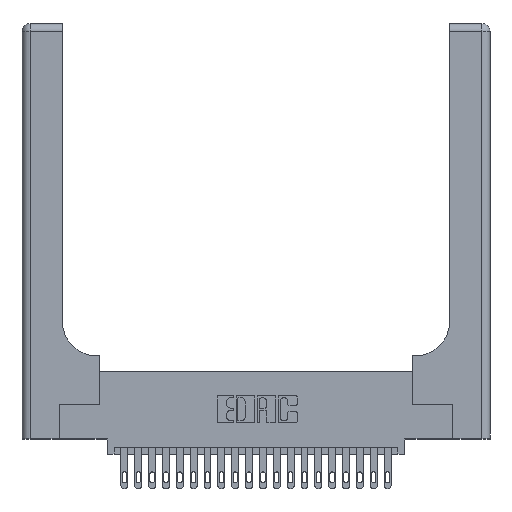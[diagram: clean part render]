
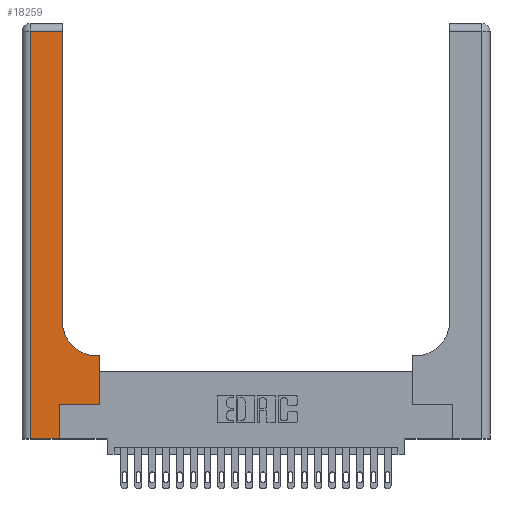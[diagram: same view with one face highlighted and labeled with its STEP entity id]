
A CAD part, top view. The second image highlights one B-rep face of the part: STEP entity #18259.
In plain terms, the highlighted planar face has unit normal (0, 0, 1).
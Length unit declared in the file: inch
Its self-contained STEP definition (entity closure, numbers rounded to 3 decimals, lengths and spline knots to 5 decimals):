
#500 = ORIENTED_EDGE ( 'NONE', *, *, #10486, .T. ) ;
#1205 = CIRCLE ( 'NONE', #1268, 0.25 ) ;
#1268 = AXIS2_PLACEMENT_3D ( 'NONE', #23259, #3258, #17698 ) ;
#1542 = EDGE_CURVE ( 'NONE', #22544, #12693, #17768, .T. ) ;
#1891 = ORIENTED_EDGE ( 'NONE', *, *, #5390, .T. ) ;
#2376 = CARTESIAN_POINT ( 'NONE',  ( 0., 0., 0.37 ) ) ;
#2495 = CARTESIAN_POINT ( 'NONE',  ( 0.06, 2.94, 0.37 ) ) ;
#2774 = DIRECTION ( 'NONE',  ( 0., 1., 0. ) ) ;
#3258 = DIRECTION ( 'NONE',  ( 0., 0., -1. ) ) ;
#3374 = ORIENTED_EDGE ( 'NONE', *, *, #15686, .T. ) ;
#3436 = CARTESIAN_POINT ( 'NONE',  ( 0.269, 0.25, 0.37 ) ) ;
#3561 = PLANE ( 'NONE',  #6685 ) ;
#4401 = DIRECTION ( 'NONE',  ( 0., 1., 0. ) ) ;
#4702 = VERTEX_POINT ( 'NONE', #19270 ) ;
#5390 = EDGE_CURVE ( 'NONE', #17954, #4702, #20363, .T. ) ;
#5890 = VECTOR ( 'NONE', #2774, 39.37008 ) ;
#6685 = AXIS2_PLACEMENT_3D ( 'NONE', #20252, #18329, #20096 ) ;
#6713 = EDGE_CURVE ( 'NONE', #21719, #17954, #14577, .T. ) ;
#7044 = EDGE_CURVE ( 'NONE', #22704, #21719, #17745, .T. ) ;
#7261 = DIRECTION ( 'NONE',  ( 1., 0., 0. ) ) ;
#7413 = DIRECTION ( 'NONE',  ( 0., 1., 0. ) ) ;
#7631 = CARTESIAN_POINT ( 'NONE',  ( 0.5415, 0.6, 0.37 ) ) ;
#8100 = VERTEX_POINT ( 'NONE', #14415 ) ;
#8225 = EDGE_CURVE ( 'NONE', #8100, #19364, #15338, .T. ) ;
#8270 = CARTESIAN_POINT ( 'NONE',  ( 0.2915, 2.94, 0.37 ) ) ;
#8557 = EDGE_LOOP ( 'NONE', ( #14860, #19888, #1891, #20230, #17797, #500, #18444, #15150, #3374 ) ) ;
#9401 = EDGE_CURVE ( 'NONE', #4702, #8100, #17921, .T. ) ;
#10427 = VECTOR ( 'NONE', #7413, 39.37008 ) ;
#10486 = EDGE_CURVE ( 'NONE', #19364, #22544, #21333, .T. ) ;
#11008 = CARTESIAN_POINT ( 'NONE',  ( 0.269, 0.25, 0.37 ) ) ;
#11228 = CARTESIAN_POINT ( 'NONE',  ( 0.5585, 0.25, 0.37 ) ) ;
#11349 = EDGE_CURVE ( 'NONE', #12693, #13190, #15800, .T. ) ;
#12320 = VECTOR ( 'NONE', #15314, 39.37008 ) ;
#12693 = VERTEX_POINT ( 'NONE', #15752 ) ;
#13190 = VERTEX_POINT ( 'NONE', #7631 ) ;
#13275 = DIRECTION ( 'NONE',  ( 1., 0., 0. ) ) ;
#13382 = VECTOR ( 'NONE', #4401, 39.37008 ) ;
#13425 = VECTOR ( 'NONE', #21799, 39.37008 ) ;
#14415 = CARTESIAN_POINT ( 'NONE',  ( 0.269, 0., 0.37 ) ) ;
#14577 = LINE ( 'NONE', #15600, #20868 ) ;
#14860 = ORIENTED_EDGE ( 'NONE', *, *, #7044, .T. ) ;
#15150 = ORIENTED_EDGE ( 'NONE', *, *, #11349, .T. ) ;
#15314 = DIRECTION ( 'NONE',  ( -1., 0., 0. ) ) ;
#15338 = LINE ( 'NONE', #20348, #10427 ) ;
#15573 = VECTOR ( 'NONE', #7261, 39.37008 ) ;
#15600 = CARTESIAN_POINT ( 'NONE',  ( 0., 2.94, 0.37 ) ) ;
#15686 = EDGE_CURVE ( 'NONE', #13190, #22704, #1205, .T. ) ;
#15752 = CARTESIAN_POINT ( 'NONE',  ( 0.5585, 0.6, 0.37 ) ) ;
#15800 = LINE ( 'NONE', #16702, #12320 ) ;
#16702 = CARTESIAN_POINT ( 'NONE',  ( 0.2915, 0.6, 0.37 ) ) ;
#17698 = DIRECTION ( 'NONE',  ( 1., 0., 0. ) ) ;
#17745 = LINE ( 'NONE', #20960, #13382 ) ;
#17768 = LINE ( 'NONE', #23183, #5890 ) ;
#17797 = ORIENTED_EDGE ( 'NONE', *, *, #8225, .T. ) ;
#17921 = LINE ( 'NONE', #2376, #19348 ) ;
#17954 = VERTEX_POINT ( 'NONE', #2495 ) ;
#18259 = ADVANCED_FACE ( 'NONE', ( #22284 ), #3561, .F. ) ;
#18329 = DIRECTION ( 'NONE',  ( 0., 0., -1. ) ) ;
#18444 = ORIENTED_EDGE ( 'NONE', *, *, #1542, .T. ) ;
#19270 = CARTESIAN_POINT ( 'NONE',  ( 0.06, 0., 0.37 ) ) ;
#19348 = VECTOR ( 'NONE', #13275, 39.37008 ) ;
#19364 = VERTEX_POINT ( 'NONE', #11008 ) ;
#19762 = CARTESIAN_POINT ( 'NONE',  ( 0.06, 3., 0.37 ) ) ;
#19783 = DIRECTION ( 'NONE',  ( -1., 0., 0. ) ) ;
#19888 = ORIENTED_EDGE ( 'NONE', *, *, #6713, .T. ) ;
#20096 = DIRECTION ( 'NONE',  ( -1., 0., 0. ) ) ;
#20230 = ORIENTED_EDGE ( 'NONE', *, *, #9401, .T. ) ;
#20252 = CARTESIAN_POINT ( 'NONE',  ( 0., 3., 0.37 ) ) ;
#20348 = CARTESIAN_POINT ( 'NONE',  ( 0.269, 0., 0.37 ) ) ;
#20363 = LINE ( 'NONE', #19762, #13425 ) ;
#20512 = CARTESIAN_POINT ( 'NONE',  ( 0.2915, 0.85, 0.37 ) ) ;
#20868 = VECTOR ( 'NONE', #19783, 39.37008 ) ;
#20960 = CARTESIAN_POINT ( 'NONE',  ( 0.2915, 3., 0.37 ) ) ;
#21333 = LINE ( 'NONE', #3436, #15573 ) ;
#21719 = VERTEX_POINT ( 'NONE', #8270 ) ;
#21799 = DIRECTION ( 'NONE',  ( 0., -1., 0. ) ) ;
#22284 = FACE_OUTER_BOUND ( 'NONE', #8557, .T. ) ;
#22544 = VERTEX_POINT ( 'NONE', #11228 ) ;
#22704 = VERTEX_POINT ( 'NONE', #20512 ) ;
#23183 = CARTESIAN_POINT ( 'NONE',  ( 0.5585, 0.25, 0.37 ) ) ;
#23259 = CARTESIAN_POINT ( 'NONE',  ( 0.5415, 0.85, 0.37 ) ) ;
